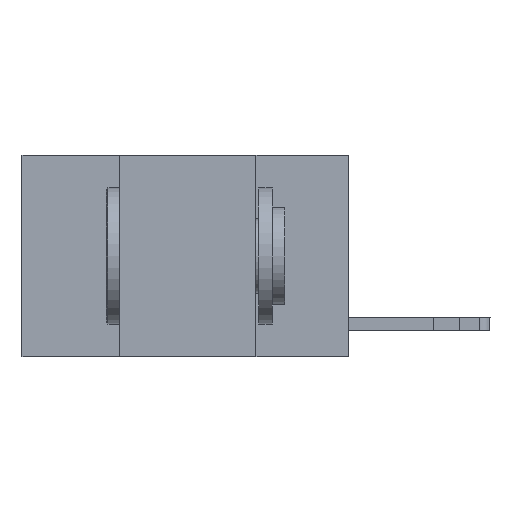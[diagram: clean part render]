
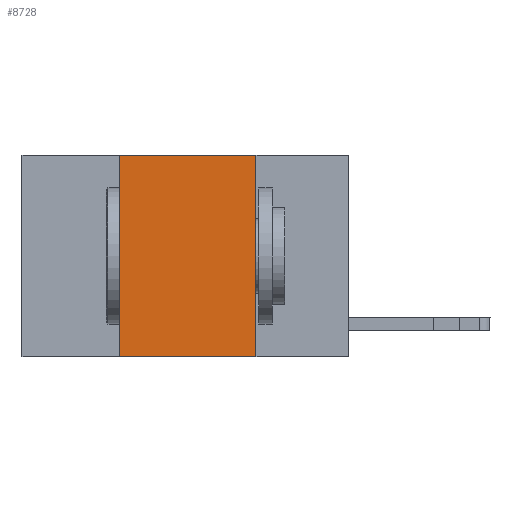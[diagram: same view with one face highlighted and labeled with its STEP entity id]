
A CAD part, left-side view. The second image highlights one B-rep face of the part: STEP entity #8728.
In plain terms, the highlighted planar face has unit normal (-1, 0, 0).
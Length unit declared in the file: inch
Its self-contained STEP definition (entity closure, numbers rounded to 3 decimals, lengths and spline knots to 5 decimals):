
#592 = VECTOR ( 'NONE', #9497, 39.37008 ) ;
#612 = VECTOR ( 'NONE', #5437, 39.37008 ) ;
#671 = LINE ( 'NONE', #3828, #592 ) ;
#1243 = LINE ( 'NONE', #5547, #12138 ) ;
#2165 = ORIENTED_EDGE ( 'NONE', *, *, #2187, .F. ) ;
#2187 = EDGE_CURVE ( 'NONE', #13898, #9544, #671, .T. ) ;
#2307 = VERTEX_POINT ( 'NONE', #4017 ) ;
#2565 = ORIENTED_EDGE ( 'NONE', *, *, #2889, .T. ) ;
#2889 = EDGE_CURVE ( 'NONE', #13898, #11407, #5346, .T. ) ;
#3828 = CARTESIAN_POINT ( 'NONE',  ( 0., 0.42, 0. ) ) ;
#4017 = CARTESIAN_POINT ( 'NONE',  ( 0., 0.17, 0. ) ) ;
#4048 = DIRECTION ( 'NONE',  ( 1., 0., 0. ) ) ;
#4578 = EDGE_LOOP ( 'NONE', ( #7147, #18297, #2165, #2565 ) ) ;
#4646 = CARTESIAN_POINT ( 'NONE',  ( 0., 0.6, 0. ) ) ;
#5346 = LINE ( 'NONE', #14607, #612 ) ;
#5437 = DIRECTION ( 'NONE',  ( 0., -1., 0. ) ) ;
#5547 = CARTESIAN_POINT ( 'NONE',  ( 0., 0.17, 0. ) ) ;
#7147 = ORIENTED_EDGE ( 'NONE', *, *, #9091, .F. ) ;
#8366 = PLANE ( 'NONE',  #16535 ) ;
#8728 = ADVANCED_FACE ( 'NONE', ( #19275 ), #8366, .F. ) ;
#9091 = EDGE_CURVE ( 'NONE', #2307, #11407, #1243, .T. ) ;
#9497 = DIRECTION ( 'NONE',  ( 0., 0., 1. ) ) ;
#9544 = VERTEX_POINT ( 'NONE', #10061 ) ;
#10035 = DIRECTION ( 'NONE',  ( 0., 0., -1. ) ) ;
#10061 = CARTESIAN_POINT ( 'NONE',  ( 0., 0.42, 0. ) ) ;
#11407 = VERTEX_POINT ( 'NONE', #14719 ) ;
#11913 = VECTOR ( 'NONE', #15070, 39.37008 ) ;
#12138 = VECTOR ( 'NONE', #14718, 39.37008 ) ;
#13443 = EDGE_CURVE ( 'NONE', #9544, #2307, #16538, .T. ) ;
#13898 = VERTEX_POINT ( 'NONE', #14919 ) ;
#14607 = CARTESIAN_POINT ( 'NONE',  ( 0., 0.6, -0.37 ) ) ;
#14718 = DIRECTION ( 'NONE',  ( 0., 0., -1. ) ) ;
#14719 = CARTESIAN_POINT ( 'NONE',  ( 0., 0.17, -0.37 ) ) ;
#14919 = CARTESIAN_POINT ( 'NONE',  ( 0., 0.42, -0.37 ) ) ;
#15070 = DIRECTION ( 'NONE',  ( 0., -1., 0. ) ) ;
#16535 = AXIS2_PLACEMENT_3D ( 'NONE', #17501, #4048, #10035 ) ;
#16538 = LINE ( 'NONE', #4646, #11913 ) ;
#17501 = CARTESIAN_POINT ( 'NONE',  ( 0., 0.6, 0. ) ) ;
#18297 = ORIENTED_EDGE ( 'NONE', *, *, #13443, .F. ) ;
#19275 = FACE_OUTER_BOUND ( 'NONE', #4578, .T. ) ;
